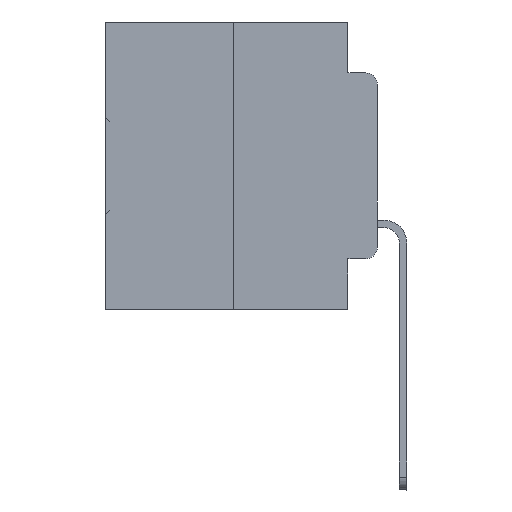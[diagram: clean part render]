
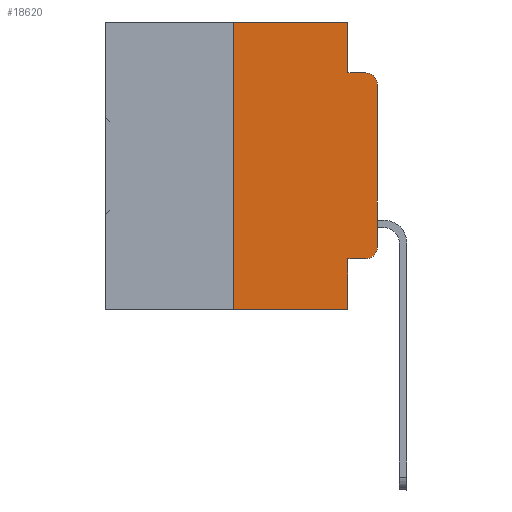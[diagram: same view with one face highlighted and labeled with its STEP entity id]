
A CAD part, left-side view. The second image highlights one B-rep face of the part: STEP entity #18620.
In plain terms, the highlighted planar face has unit normal (-1, 0, 0).
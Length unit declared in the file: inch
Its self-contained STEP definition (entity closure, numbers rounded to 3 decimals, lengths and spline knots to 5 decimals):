
#1144 = VECTOR ( 'NONE', #20403, 39.37008 ) ;
#1504 = LINE ( 'NONE', #19429, #7093 ) ;
#2324 = EDGE_CURVE ( 'NONE', #5261, #31363, #1504, .T. ) ;
#2522 = EDGE_CURVE ( 'NONE', #12290, #9307, #15552, .T. ) ;
#2543 = ORIENTED_EDGE ( 'NONE', *, *, #20265, .T. ) ;
#2671 = CARTESIAN_POINT ( 'NONE',  ( 0., 0.02, -0.1085 ) ) ;
#3326 = DIRECTION ( 'NONE',  ( 0., -1., 0. ) ) ;
#3512 = CARTESIAN_POINT ( 'NONE',  ( 0., 0.473, 0. ) ) ;
#4278 = CARTESIAN_POINT ( 'NONE',  ( 0., 0., -0.3915 ) ) ;
#4386 = DIRECTION ( 'NONE',  ( 0., -1., 0. ) ) ;
#4699 = ORIENTED_EDGE ( 'NONE', *, *, #30233, .F. ) ;
#5261 = VERTEX_POINT ( 'NONE', #4278 ) ;
#5512 = DIRECTION ( 'NONE',  ( 0., 0., -1. ) ) ;
#5797 = VERTEX_POINT ( 'NONE', #17634 ) ;
#5850 = EDGE_CURVE ( 'NONE', #28084, #12290, #22151, .T. ) ;
#6393 = DIRECTION ( 'NONE',  ( 0., 0., 1. ) ) ;
#6800 = VECTOR ( 'NONE', #5512, 39.37008 ) ;
#6813 = ORIENTED_EDGE ( 'NONE', *, *, #2522, .F. ) ;
#7093 = VECTOR ( 'NONE', #6393, 39.37008 ) ;
#8618 = ORIENTED_EDGE ( 'NONE', *, *, #15257, .T. ) ;
#9307 = VERTEX_POINT ( 'NONE', #15283 ) ;
#9561 = CARTESIAN_POINT ( 'NONE',  ( 0., 0.051, -0.5 ) ) ;
#10808 = CARTESIAN_POINT ( 'NONE',  ( 0., 0.051, -0.0885 ) ) ;
#11388 = DIRECTION ( 'NONE',  ( -1., 0., 0. ) ) ;
#11456 = VERTEX_POINT ( 'NONE', #12652 ) ;
#11480 = CARTESIAN_POINT ( 'NONE',  ( 0., 0., -0.1085 ) ) ;
#11633 = LINE ( 'NONE', #33310, #34639 ) ;
#12290 = VERTEX_POINT ( 'NONE', #10808 ) ;
#12393 = VECTOR ( 'NONE', #31567, 39.37008 ) ;
#12652 = CARTESIAN_POINT ( 'NONE',  ( 0., 0.25, -0.5 ) ) ;
#12778 = CARTESIAN_POINT ( 'NONE',  ( 0., 0.051, -0.0885 ) ) ;
#13594 = ORIENTED_EDGE ( 'NONE', *, *, #32937, .F. ) ;
#14101 = CARTESIAN_POINT ( 'NONE',  ( 0., 0.473, 0. ) ) ;
#14240 = LINE ( 'NONE', #14101, #24103 ) ;
#14856 = AXIS2_PLACEMENT_3D ( 'NONE', #3512, #23005, #20377 ) ;
#14960 = CARTESIAN_POINT ( 'NONE',  ( 0., 0.051, 0. ) ) ;
#15257 = EDGE_CURVE ( 'NONE', #31363, #9307, #27345, .T. ) ;
#15283 = CARTESIAN_POINT ( 'NONE',  ( 0., 0.02, -0.0885 ) ) ;
#15478 = AXIS2_PLACEMENT_3D ( 'NONE', #2671, #16300, #33129 ) ;
#15552 = LINE ( 'NONE', #12778, #15595 ) ;
#15595 = VECTOR ( 'NONE', #4386, 39.37008 ) ;
#15954 = CARTESIAN_POINT ( 'NONE',  ( 0., 0.02, -0.4115 ) ) ;
#16300 = DIRECTION ( 'NONE',  ( -1., 0., 0. ) ) ;
#16383 = VERTEX_POINT ( 'NONE', #9561 ) ;
#17130 = PLANE ( 'NONE',  #14856 ) ;
#17513 = CARTESIAN_POINT ( 'NONE',  ( 0., 0.051, 0. ) ) ;
#17634 = CARTESIAN_POINT ( 'NONE',  ( 0., 0.051, -0.4115 ) ) ;
#18620 = ADVANCED_FACE ( 'NONE', ( #25022 ), #17130, .F. ) ;
#19137 = DIRECTION ( 'NONE',  ( 0., 0., -1. ) ) ;
#19429 = CARTESIAN_POINT ( 'NONE',  ( 0., 0., 0. ) ) ;
#19787 = AXIS2_PLACEMENT_3D ( 'NONE', #24911, #11388, #19137 ) ;
#20265 = EDGE_CURVE ( 'NONE', #5797, #31867, #11633, .T. ) ;
#20377 = DIRECTION ( 'NONE',  ( 0., 0., -1. ) ) ;
#20403 = DIRECTION ( 'NONE',  ( 0., 0., -1. ) ) ;
#22151 = LINE ( 'NONE', #17513, #1144 ) ;
#22603 = DIRECTION ( 'NONE',  ( 0., -1., 0. ) ) ;
#23005 = DIRECTION ( 'NONE',  ( 1., 0., 0. ) ) ;
#23092 = EDGE_CURVE ( 'NONE', #31867, #5261, #33502, .T. ) ;
#24103 = VECTOR ( 'NONE', #3326, 39.37008 ) ;
#24338 = ORIENTED_EDGE ( 'NONE', *, *, #29972, .T. ) ;
#24455 = CARTESIAN_POINT ( 'NONE',  ( 0., 0.25, 0. ) ) ;
#24911 = CARTESIAN_POINT ( 'NONE',  ( 0., 0.02, -0.3915 ) ) ;
#25022 = FACE_OUTER_BOUND ( 'NONE', #33413, .T. ) ;
#25566 = VERTEX_POINT ( 'NONE', #24455 ) ;
#27092 = LINE ( 'NONE', #28922, #30068 ) ;
#27345 = CIRCLE ( 'NONE', #15478, 0.02 ) ;
#27379 = CARTESIAN_POINT ( 'NONE',  ( 0., 0.051, 0. ) ) ;
#27818 = ORIENTED_EDGE ( 'NONE', *, *, #33243, .F. ) ;
#28084 = VERTEX_POINT ( 'NONE', #14960 ) ;
#28701 = CARTESIAN_POINT ( 'NONE',  ( 0., 0.473, -0.5 ) ) ;
#28922 = CARTESIAN_POINT ( 'NONE',  ( 0., 0.25, 0. ) ) ;
#29972 = EDGE_CURVE ( 'NONE', #11456, #16383, #33295, .T. ) ;
#30068 = VECTOR ( 'NONE', #34253, 39.37008 ) ;
#30233 = EDGE_CURVE ( 'NONE', #5797, #16383, #34098, .T. ) ;
#31157 = ORIENTED_EDGE ( 'NONE', *, *, #5850, .F. ) ;
#31363 = VERTEX_POINT ( 'NONE', #11480 ) ;
#31567 = DIRECTION ( 'NONE',  ( 0., -1., 0. ) ) ;
#31867 = VERTEX_POINT ( 'NONE', #15954 ) ;
#32937 = EDGE_CURVE ( 'NONE', #11456, #25566, #27092, .T. ) ;
#33129 = DIRECTION ( 'NONE',  ( 0., 0., -1. ) ) ;
#33243 = EDGE_CURVE ( 'NONE', #25566, #28084, #14240, .T. ) ;
#33295 = LINE ( 'NONE', #28701, #12393 ) ;
#33305 = ORIENTED_EDGE ( 'NONE', *, *, #23092, .T. ) ;
#33310 = CARTESIAN_POINT ( 'NONE',  ( 0., 0.051, -0.4115 ) ) ;
#33413 = EDGE_LOOP ( 'NONE', ( #34117, #8618, #6813, #31157, #27818, #13594, #24338, #4699, #2543, #33305 ) ) ;
#33502 = CIRCLE ( 'NONE', #19787, 0.02 ) ;
#34098 = LINE ( 'NONE', #27379, #6800 ) ;
#34117 = ORIENTED_EDGE ( 'NONE', *, *, #2324, .T. ) ;
#34253 = DIRECTION ( 'NONE',  ( 0., 0., 1. ) ) ;
#34639 = VECTOR ( 'NONE', #22603, 39.37008 ) ;
